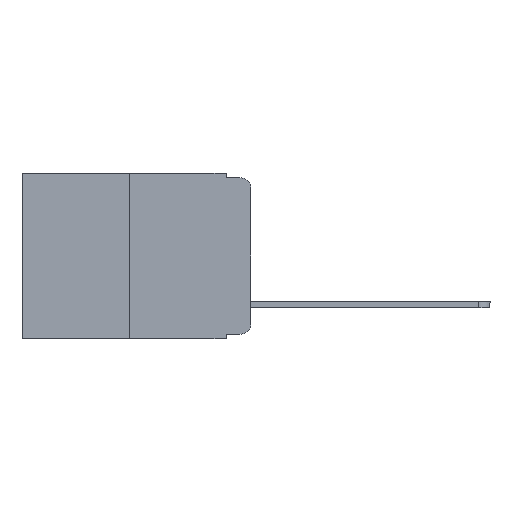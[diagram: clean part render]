
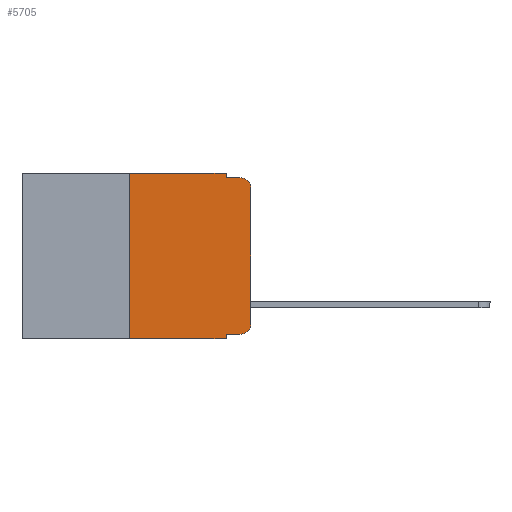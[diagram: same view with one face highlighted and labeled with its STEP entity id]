
A CAD part, left-side view. The second image highlights one B-rep face of the part: STEP entity #5705.
In plain terms, the highlighted planar face has unit normal (-1, 0, 0).
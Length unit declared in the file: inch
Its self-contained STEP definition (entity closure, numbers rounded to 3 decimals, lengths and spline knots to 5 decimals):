
#14 = EDGE_CURVE ( 'NONE', #853, #6472, #11636, .T. ) ;
#92 = DIRECTION ( 'NONE',  ( -1., 0., 0. ) ) ;
#178 = EDGE_CURVE ( 'NONE', #4861, #1639, #9406, .T. ) ;
#184 = DIRECTION ( 'NONE',  ( 0., 0., -1. ) ) ;
#477 = ORIENTED_EDGE ( 'NONE', *, *, #9027, .T. ) ;
#608 = VERTEX_POINT ( 'NONE', #623 ) ;
#623 = CARTESIAN_POINT ( 'NONE',  ( 0., 0.02, -0.333 ) ) ;
#734 = DIRECTION ( 'NONE',  ( 0., 0., -1. ) ) ;
#853 = VERTEX_POINT ( 'NONE', #4695 ) ;
#890 = CARTESIAN_POINT ( 'NONE',  ( 0., 0.051, -0.01 ) ) ;
#932 = LINE ( 'NONE', #3978, #9174 ) ;
#1030 = EDGE_CURVE ( 'NONE', #3443, #11727, #3296, .T. ) ;
#1116 = ORIENTED_EDGE ( 'NONE', *, *, #8422, .T. ) ;
#1146 = DIRECTION ( 'NONE',  ( 1., 0., 0. ) ) ;
#1367 = AXIS2_PLACEMENT_3D ( 'NONE', #6137, #1146, #184 ) ;
#1378 = CIRCLE ( 'NONE', #6628, 0.02 ) ;
#1639 = VERTEX_POINT ( 'NONE', #9835 ) ;
#2082 = LINE ( 'NONE', #12252, #5981 ) ;
#2119 = CARTESIAN_POINT ( 'NONE',  ( 0., 0.051, -0.343 ) ) ;
#2136 = PLANE ( 'NONE',  #1367 ) ;
#2488 = CARTESIAN_POINT ( 'NONE',  ( 0., 0., 0. ) ) ;
#2669 = ORIENTED_EDGE ( 'NONE', *, *, #14, .F. ) ;
#2736 = DIRECTION ( 'NONE',  ( 0., 0., 1. ) ) ;
#3271 = VECTOR ( 'NONE', #4179, 39.37008 ) ;
#3296 = CIRCLE ( 'NONE', #4978, 0.02 ) ;
#3442 = ORIENTED_EDGE ( 'NONE', *, *, #10005, .F. ) ;
#3443 = VERTEX_POINT ( 'NONE', #10586 ) ;
#3978 = CARTESIAN_POINT ( 'NONE',  ( 0., 0.051, 0. ) ) ;
#4049 = ORIENTED_EDGE ( 'NONE', *, *, #10325, .F. ) ;
#4146 = VERTEX_POINT ( 'NONE', #2119 ) ;
#4179 = DIRECTION ( 'NONE',  ( 0., -1., 0. ) ) ;
#4244 = FACE_OUTER_BOUND ( 'NONE', #6048, .T. ) ;
#4284 = VECTOR ( 'NONE', #12618, 39.37008 ) ;
#4550 = CARTESIAN_POINT ( 'NONE',  ( 0., 0.02, -0.313 ) ) ;
#4658 = ORIENTED_EDGE ( 'NONE', *, *, #5875, .T. ) ;
#4692 = LINE ( 'NONE', #8674, #9761 ) ;
#4695 = CARTESIAN_POINT ( 'NONE',  ( 0., 0.25, -0.343 ) ) ;
#4699 = CARTESIAN_POINT ( 'NONE',  ( 0., 0.25, 0. ) ) ;
#4861 = VERTEX_POINT ( 'NONE', #9360 ) ;
#4906 = DIRECTION ( 'NONE',  ( 0., -1., 0. ) ) ;
#4945 = DIRECTION ( 'NONE',  ( 0., 0., -1. ) ) ;
#4978 = AXIS2_PLACEMENT_3D ( 'NONE', #5142, #92, #4945 ) ;
#5142 = CARTESIAN_POINT ( 'NONE',  ( 0., 0.02, -0.03 ) ) ;
#5593 = CARTESIAN_POINT ( 'NONE',  ( 0., 0.051, 0. ) ) ;
#5705 = ADVANCED_FACE ( 'NONE', ( #4244 ), #2136, .F. ) ;
#5725 = DIRECTION ( 'NONE',  ( 0., -1., 0. ) ) ;
#5741 = ORIENTED_EDGE ( 'NONE', *, *, #1030, .T. ) ;
#5809 = VERTEX_POINT ( 'NONE', #10740 ) ;
#5875 = EDGE_CURVE ( 'NONE', #853, #4146, #10209, .T. ) ;
#5981 = VECTOR ( 'NONE', #10222, 39.37008 ) ;
#6048 = EDGE_LOOP ( 'NONE', ( #1116, #5741, #3442, #12843, #6997, #2669, #4658, #4049, #477, #7546 ) ) ;
#6074 = EDGE_CURVE ( 'NONE', #6472, #4861, #4692, .T. ) ;
#6137 = CARTESIAN_POINT ( 'NONE',  ( 0., 0.473, 0. ) ) ;
#6472 = VERTEX_POINT ( 'NONE', #6741 ) ;
#6592 = VECTOR ( 'NONE', #2736, 39.37008 ) ;
#6607 = DIRECTION ( 'NONE',  ( 0., 0., 1. ) ) ;
#6628 = AXIS2_PLACEMENT_3D ( 'NONE', #4550, #8598, #734 ) ;
#6741 = CARTESIAN_POINT ( 'NONE',  ( 0., 0.25, 0. ) ) ;
#6909 = DIRECTION ( 'NONE',  ( 0., 0., -1. ) ) ;
#6997 = ORIENTED_EDGE ( 'NONE', *, *, #6074, .F. ) ;
#7001 = CARTESIAN_POINT ( 'NONE',  ( 0., 0., -0.313 ) ) ;
#7184 = EDGE_CURVE ( 'NONE', #608, #12401, #1378, .T. ) ;
#7295 = CARTESIAN_POINT ( 'NONE',  ( 0., 0.473, -0.343 ) ) ;
#7546 = ORIENTED_EDGE ( 'NONE', *, *, #7184, .T. ) ;
#8295 = VECTOR ( 'NONE', #4906, 39.37008 ) ;
#8422 = EDGE_CURVE ( 'NONE', #12401, #3443, #11468, .T. ) ;
#8598 = DIRECTION ( 'NONE',  ( -1., 0., 0. ) ) ;
#8674 = CARTESIAN_POINT ( 'NONE',  ( 0., 0.473, 0. ) ) ;
#9027 = EDGE_CURVE ( 'NONE', #5809, #608, #2082, .T. ) ;
#9174 = VECTOR ( 'NONE', #6909, 39.37008 ) ;
#9273 = CARTESIAN_POINT ( 'NONE',  ( 0., 0.02, -0.01 ) ) ;
#9360 = CARTESIAN_POINT ( 'NONE',  ( 0., 0.051, 0. ) ) ;
#9406 = LINE ( 'NONE', #5593, #4284 ) ;
#9761 = VECTOR ( 'NONE', #5725, 39.37008 ) ;
#9835 = CARTESIAN_POINT ( 'NONE',  ( 0., 0.051, -0.01 ) ) ;
#9883 = LINE ( 'NONE', #890, #8295 ) ;
#10005 = EDGE_CURVE ( 'NONE', #1639, #11727, #9883, .T. ) ;
#10209 = LINE ( 'NONE', #7295, #3271 ) ;
#10222 = DIRECTION ( 'NONE',  ( 0., -1., 0. ) ) ;
#10325 = EDGE_CURVE ( 'NONE', #5809, #4146, #932, .T. ) ;
#10586 = CARTESIAN_POINT ( 'NONE',  ( 0., 0., -0.03 ) ) ;
#10740 = CARTESIAN_POINT ( 'NONE',  ( 0., 0.051, -0.333 ) ) ;
#10872 = VECTOR ( 'NONE', #6607, 39.37008 ) ;
#11468 = LINE ( 'NONE', #2488, #10872 ) ;
#11636 = LINE ( 'NONE', #4699, #6592 ) ;
#11727 = VERTEX_POINT ( 'NONE', #9273 ) ;
#12252 = CARTESIAN_POINT ( 'NONE',  ( 0., 0.051, -0.333 ) ) ;
#12401 = VERTEX_POINT ( 'NONE', #7001 ) ;
#12618 = DIRECTION ( 'NONE',  ( 0., 0., -1. ) ) ;
#12843 = ORIENTED_EDGE ( 'NONE', *, *, #178, .F. ) ;
